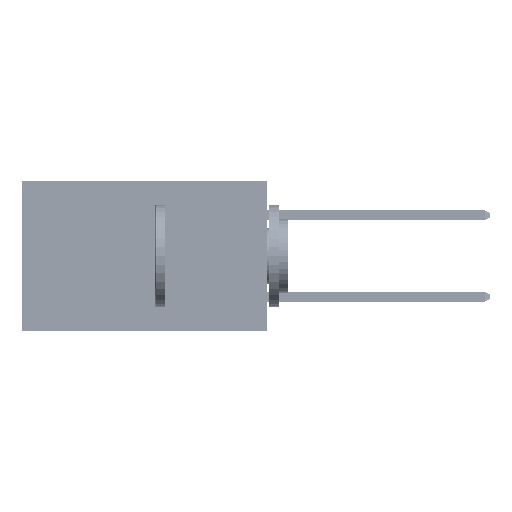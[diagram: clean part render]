
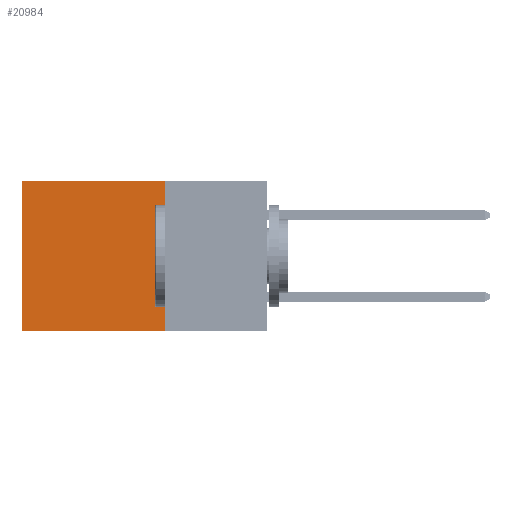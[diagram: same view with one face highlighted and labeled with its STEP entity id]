
A CAD part, left-side view. The second image highlights one B-rep face of the part: STEP entity #20984.
In plain terms, the highlighted planar face has unit normal (-1, 0, 0).
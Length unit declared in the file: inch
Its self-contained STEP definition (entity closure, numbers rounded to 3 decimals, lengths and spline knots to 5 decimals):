
#91 = DIRECTION ( 'NONE',  ( 0., 1., 0. ) ) ;
#559 = LINE ( 'NONE', #47526, #36932 ) ;
#736 = ORIENTED_EDGE ( 'NONE', *, *, #25763, .F. ) ;
#3981 = ORIENTED_EDGE ( 'NONE', *, *, #5659, .T. ) ;
#4159 = VERTEX_POINT ( 'NONE', #28783 ) ;
#4609 = CARTESIAN_POINT ( 'NONE',  ( 0.2875, 0.6, 0. ) ) ;
#5659 = EDGE_CURVE ( 'NONE', #4159, #8754, #14395, .T. ) ;
#7472 = AXIS2_PLACEMENT_3D ( 'NONE', #26406, #33313, #33806 ) ;
#8754 = VERTEX_POINT ( 'NONE', #4609 ) ;
#9597 = CARTESIAN_POINT ( 'NONE',  ( 0.2875, 0.6, -0.37 ) ) ;
#14395 = LINE ( 'NONE', #41269, #36139 ) ;
#14435 = DIRECTION ( 'NONE',  ( 0., 0., -1. ) ) ;
#14734 = ORIENTED_EDGE ( 'NONE', *, *, #29389, .F. ) ;
#17798 = VECTOR ( 'NONE', #14435, 39.37008 ) ;
#19143 = CARTESIAN_POINT ( 'NONE',  ( 0.2875, 0.25, -0.37 ) ) ;
#19392 = DIRECTION ( 'NONE',  ( 0., 0., -1. ) ) ;
#19554 = CARTESIAN_POINT ( 'NONE',  ( 0.2875, 0.25, 0. ) ) ;
#20984 = ADVANCED_FACE ( 'NONE', ( #41980 ), #26243, .F. ) ;
#22274 = CARTESIAN_POINT ( 'NONE',  ( 0.2875, 0.6, 0. ) ) ;
#25657 = VECTOR ( 'NONE', #19392, 39.37008 ) ;
#25763 = EDGE_CURVE ( 'NONE', #32046, #26316, #559, .T. ) ;
#26243 = PLANE ( 'NONE',  #7472 ) ;
#26316 = VERTEX_POINT ( 'NONE', #9597 ) ;
#26406 = CARTESIAN_POINT ( 'NONE',  ( 0.2875, 0.25, 0. ) ) ;
#28783 = CARTESIAN_POINT ( 'NONE',  ( 0.2875, 0.25, 0. ) ) ;
#29389 = EDGE_CURVE ( 'NONE', #4159, #32046, #46286, .T. ) ;
#31757 = EDGE_CURVE ( 'NONE', #8754, #26316, #34235, .T. ) ;
#32046 = VERTEX_POINT ( 'NONE', #19143 ) ;
#33313 = DIRECTION ( 'NONE',  ( 1., 0., 0. ) ) ;
#33806 = DIRECTION ( 'NONE',  ( 0., 0., -1. ) ) ;
#34235 = LINE ( 'NONE', #22274, #17798 ) ;
#36139 = VECTOR ( 'NONE', #91, 39.37008 ) ;
#36423 = EDGE_LOOP ( 'NONE', ( #47847, #736, #14734, #3981 ) ) ;
#36932 = VECTOR ( 'NONE', #40308, 39.37008 ) ;
#40308 = DIRECTION ( 'NONE',  ( 0., 1., 0. ) ) ;
#41269 = CARTESIAN_POINT ( 'NONE',  ( 0.2875, 0.25, 0. ) ) ;
#41980 = FACE_OUTER_BOUND ( 'NONE', #36423, .T. ) ;
#46286 = LINE ( 'NONE', #19554, #25657 ) ;
#47526 = CARTESIAN_POINT ( 'NONE',  ( 0.2875, 0.25, -0.37 ) ) ;
#47847 = ORIENTED_EDGE ( 'NONE', *, *, #31757, .T. ) ;
